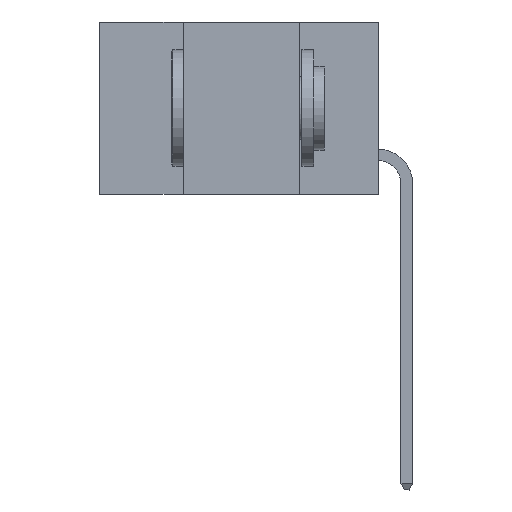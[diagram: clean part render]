
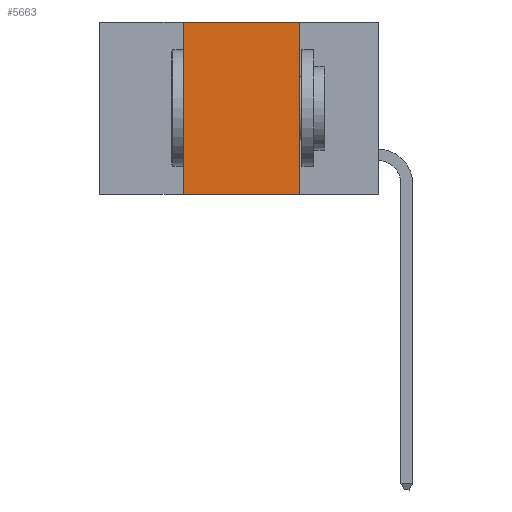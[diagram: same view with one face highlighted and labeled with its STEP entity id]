
A CAD part, left-side view. The second image highlights one B-rep face of the part: STEP entity #5663.
In plain terms, the highlighted planar face has unit normal (-1, 0, 0).
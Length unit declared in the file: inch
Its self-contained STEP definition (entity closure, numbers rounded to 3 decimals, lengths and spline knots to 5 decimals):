
#444 = VECTOR ( 'NONE', #9129, 39.37008 ) ;
#563 = DIRECTION ( 'NONE',  ( 1., 0., 0. ) ) ;
#661 = DIRECTION ( 'NONE',  ( 0., 0., -1. ) ) ;
#752 = EDGE_CURVE ( 'NONE', #19423, #18149, #14902, .T. ) ;
#754 = CARTESIAN_POINT ( 'NONE',  ( 0., 0.42, 0. ) ) ;
#1339 = CARTESIAN_POINT ( 'NONE',  ( 0., 0.17, 0. ) ) ;
#3307 = EDGE_CURVE ( 'NONE', #15173, #13468, #23882, .T. ) ;
#4196 = CARTESIAN_POINT ( 'NONE',  ( 0., 0.17, -0.37 ) ) ;
#5000 = LINE ( 'NONE', #754, #18729 ) ;
#5222 = CARTESIAN_POINT ( 'NONE',  ( 0., 0.6, 0. ) ) ;
#5663 = ADVANCED_FACE ( 'NONE', ( #24091 ), #29172, .F. ) ;
#6521 = EDGE_LOOP ( 'NONE', ( #28486, #10688, #16161, #29758 ) ) ;
#6652 = CARTESIAN_POINT ( 'NONE',  ( 0., 0.17, 0. ) ) ;
#9129 = DIRECTION ( 'NONE',  ( 0., 0., -1. ) ) ;
#10688 = ORIENTED_EDGE ( 'NONE', *, *, #3307, .F. ) ;
#12426 = VECTOR ( 'NONE', #23088, 39.37008 ) ;
#13468 = VERTEX_POINT ( 'NONE', #1339 ) ;
#13661 = CARTESIAN_POINT ( 'NONE',  ( 0., 0.6, -0.37 ) ) ;
#14902 = LINE ( 'NONE', #13661, #17102 ) ;
#15173 = VERTEX_POINT ( 'NONE', #22396 ) ;
#16161 = ORIENTED_EDGE ( 'NONE', *, *, #20567, .F. ) ;
#17102 = VECTOR ( 'NONE', #30220, 39.37008 ) ;
#18149 = VERTEX_POINT ( 'NONE', #4196 ) ;
#18190 = AXIS2_PLACEMENT_3D ( 'NONE', #5222, #563, #661 ) ;
#18729 = VECTOR ( 'NONE', #22384, 39.37008 ) ;
#19423 = VERTEX_POINT ( 'NONE', #26823 ) ;
#20567 = EDGE_CURVE ( 'NONE', #19423, #15173, #5000, .T. ) ;
#22384 = DIRECTION ( 'NONE',  ( 0., 0., 1. ) ) ;
#22396 = CARTESIAN_POINT ( 'NONE',  ( 0., 0.42, 0. ) ) ;
#22587 = CARTESIAN_POINT ( 'NONE',  ( 0., 0.6, 0. ) ) ;
#22767 = LINE ( 'NONE', #6652, #444 ) ;
#23088 = DIRECTION ( 'NONE',  ( 0., -1., 0. ) ) ;
#23882 = LINE ( 'NONE', #22587, #12426 ) ;
#24091 = FACE_OUTER_BOUND ( 'NONE', #6521, .T. ) ;
#24548 = EDGE_CURVE ( 'NONE', #13468, #18149, #22767, .T. ) ;
#26823 = CARTESIAN_POINT ( 'NONE',  ( 0., 0.42, -0.37 ) ) ;
#28486 = ORIENTED_EDGE ( 'NONE', *, *, #24548, .F. ) ;
#29172 = PLANE ( 'NONE',  #18190 ) ;
#29758 = ORIENTED_EDGE ( 'NONE', *, *, #752, .T. ) ;
#30220 = DIRECTION ( 'NONE',  ( 0., -1., 0. ) ) ;
